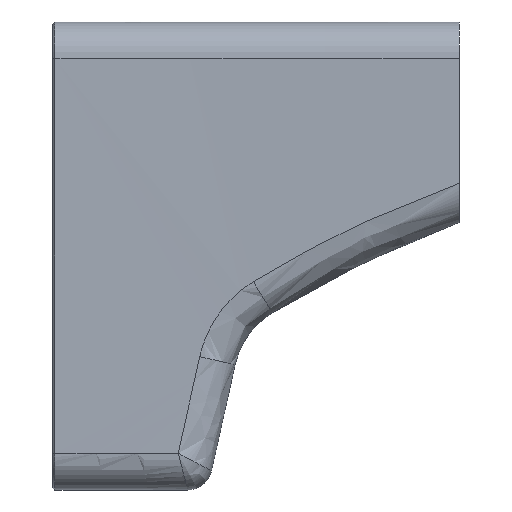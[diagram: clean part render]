
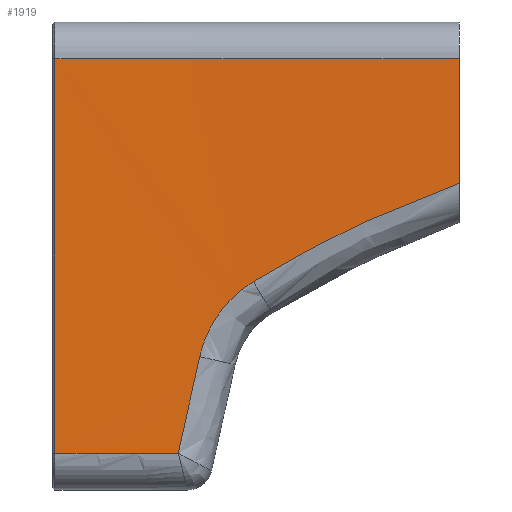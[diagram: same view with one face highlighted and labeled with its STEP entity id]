
A CAD part, left-side view. The second image highlights one B-rep face of the part: STEP entity #1919.
In plain terms, the highlighted cylindrical face has radius 3182.51 mm (diameter 6365.01 mm), a partial arc.
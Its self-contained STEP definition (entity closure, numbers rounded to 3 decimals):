
#21=ELLIPSE('',#2073,14630.042,3182.507);
#29=CYLINDRICAL_SURFACE('',#2071,3182.507);
#74=LINE('',#4348,#173);
#91=LINE('',#4991,#190);
#173=VECTOR('',#2333,10.);
#190=VECTOR('',#2368,10.);
#379=FACE_OUTER_BOUND('',#516,.T.);
#516=EDGE_LOOP('',(#1457,#1458,#1459,#1460,#1461,#1462,#1463));
#668=B_SPLINE_CURVE_WITH_KNOTS('',3,(#4981,#4982,#4983,#4984,#4985),
 .UNSPECIFIED.,.F.,.F.,(4,1,4),(0.,0.999,2.331),
 .UNSPECIFIED.);
#669=B_SPLINE_CURVE_WITH_KNOTS('',3,(#4987,#4988,#4989,#4990),
 .UNSPECIFIED.,.F.,.F.,(4,4),(0.967,6.603),
 .UNSPECIFIED.);
#719=CIRCLE('',#2069,3182.507);
#721=CIRCLE('',#2072,3182.507);
#847=VERTEX_POINT('',#4341);
#850=VERTEX_POINT('',#4346);
#871=VERTEX_POINT('',#4953);
#873=VERTEX_POINT('',#4976);
#874=VERTEX_POINT('',#4978);
#875=VERTEX_POINT('',#4980);
#876=VERTEX_POINT('',#4986);
#1050=EDGE_CURVE('',#850,#847,#74,.T.);
#1083=EDGE_CURVE('',#847,#871,#719,.T.);
#1086=EDGE_CURVE('',#873,#850,#721,.T.);
#1087=EDGE_CURVE('',#874,#873,#21,.T.);
#1088=EDGE_CURVE('',#875,#874,#668,.T.);
#1089=EDGE_CURVE('',#876,#875,#669,.T.);
#1090=EDGE_CURVE('',#876,#871,#91,.T.);
#1457=ORIENTED_EDGE('',*,*,#1050,.F.);
#1458=ORIENTED_EDGE('',*,*,#1086,.F.);
#1459=ORIENTED_EDGE('',*,*,#1087,.F.);
#1460=ORIENTED_EDGE('',*,*,#1088,.F.);
#1461=ORIENTED_EDGE('',*,*,#1089,.F.);
#1462=ORIENTED_EDGE('',*,*,#1090,.T.);
#1463=ORIENTED_EDGE('',*,*,#1083,.F.);
#1919=ADVANCED_FACE('',(#379),#29,.F.);
#2069=AXIS2_PLACEMENT_3D('',#4954,#2358,#2359);
#2071=AXIS2_PLACEMENT_3D('',#4975,#2362,#2363);
#2072=AXIS2_PLACEMENT_3D('',#4977,#2364,#2365);
#2073=AXIS2_PLACEMENT_3D('',#4979,#2366,#2367);
#2333=DIRECTION('',(0.,0.,1.));
#2358=DIRECTION('center_axis',(0.,0.,-1.));
#2359=DIRECTION('ref_axis',(1.,0.004,0.));
#2362=DIRECTION('center_axis',(0.,0.,-1.));
#2363=DIRECTION('ref_axis',(0.999,-0.041,0.));
#2364=DIRECTION('center_axis',(0.,0.,1.));
#2365=DIRECTION('ref_axis',(1.,0.015,0.));
#2366=DIRECTION('center_axis',(0.,0.976,
0.218));
#2367=DIRECTION('ref_axis',(0.,0.218,-0.976));
#2368=DIRECTION('',(0.,0.,1.));
#4341=CARTESIAN_POINT('',(0.589,399.4,-129.588));
#4346=CARTESIAN_POINT('',(0.589,399.4,-226.588));
#4348=CARTESIAN_POINT('',(0.589,399.4,-108.588));
#4953=CARTESIAN_POINT('',(0.953,300.,-129.588));
#4954=CARTESIAN_POINT('Origin',(-3181.326,338.055,-129.588));
#4975=CARTESIAN_POINT('Origin',(-3181.326,338.055,-108.588));
#4976=CARTESIAN_POINT('',(1.029,369.123,-226.588));
#4977=CARTESIAN_POINT('Origin',(-3181.326,338.055,-226.588));
#4978=CARTESIAN_POINT('',(1.076,363.826,-202.825));
#4979=CARTESIAN_POINT('Origin',(-3181.326,338.055,-87.191));
#4980=CARTESIAN_POINT('',(1.156,350.652,-184.385));
#4981=CARTESIAN_POINT('Ctrl Pts',(1.156,350.652,-184.385));
#4982=CARTESIAN_POINT('Ctrl Pts',(1.145,353.487,-186.118));
#4983=CARTESIAN_POINT('Ctrl Pts',(1.112,359.404,-191.313));
#4984=CARTESIAN_POINT('Ctrl Pts',(1.084,362.861,-198.492));
#4985=CARTESIAN_POINT('Ctrl Pts',(1.076,363.826,-202.825));
#4986=CARTESIAN_POINT('',(0.953,300.,-160.194));
#4987=CARTESIAN_POINT('Ctrl Pts',(0.953,300.,-160.194));
#4988=CARTESIAN_POINT('Ctrl Pts',(1.164,317.65,-166.489));
#4989=CARTESIAN_POINT('Ctrl Pts',(1.219,334.654,-174.61));
#4990=CARTESIAN_POINT('Ctrl Pts',(1.156,350.652,-184.385));
#4991=CARTESIAN_POINT('',(0.953,300.,-108.588));
